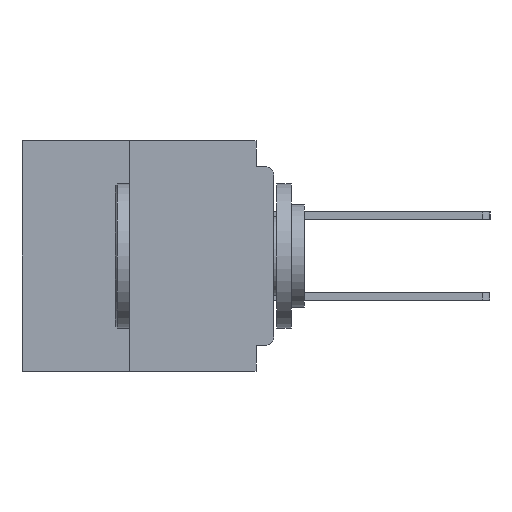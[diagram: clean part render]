
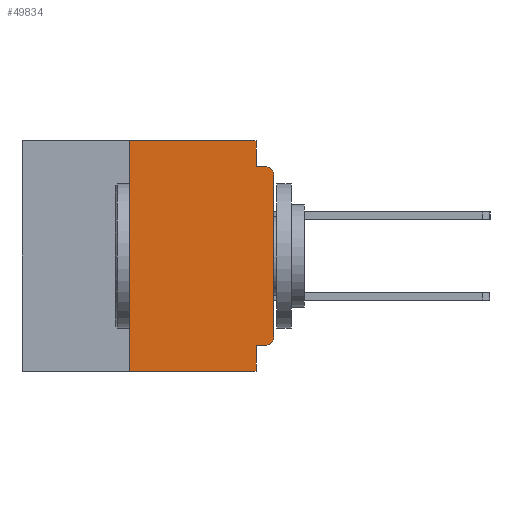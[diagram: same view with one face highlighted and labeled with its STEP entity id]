
A CAD part, left-side view. The second image highlights one B-rep face of the part: STEP entity #49834.
In plain terms, the highlighted planar face has unit normal (-1, 0, 0).
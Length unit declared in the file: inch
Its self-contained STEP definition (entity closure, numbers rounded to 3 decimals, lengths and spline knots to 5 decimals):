
#256 = CARTESIAN_POINT ( 'NONE',  ( 0., 0.031, -0.4 ) ) ;
#563 = LINE ( 'NONE', #10025, #61828 ) ;
#2432 = VECTOR ( 'NONE', #19850, 39.37008 ) ;
#3937 = LINE ( 'NONE', #24716, #2432 ) ;
#4308 = EDGE_CURVE ( 'NONE', #11964, #53646, #60278, .T. ) ;
#4399 = AXIS2_PLACEMENT_3D ( 'NONE', #24030, #57806, #28901 ) ;
#4649 = ORIENTED_EDGE ( 'NONE', *, *, #8739, .F. ) ;
#5130 = DIRECTION ( 'NONE',  ( 0., 1., 0. ) ) ;
#6956 = LINE ( 'NONE', #42299, #56839 ) ;
#6990 = CIRCLE ( 'NONE', #42177, 0.015 ) ;
#8519 = EDGE_CURVE ( 'NONE', #20073, #9102, #41814, .T. ) ;
#8619 = ORIENTED_EDGE ( 'NONE', *, *, #49815, .F. ) ;
#8739 = EDGE_CURVE ( 'NONE', #57338, #20073, #3937, .T. ) ;
#9102 = VERTEX_POINT ( 'NONE', #18107 ) ;
#9490 = DIRECTION ( 'NONE',  ( -1., 0., 0. ) ) ;
#10025 = CARTESIAN_POINT ( 'NONE',  ( 0., 0., -0.355 ) ) ;
#11177 = VERTEX_POINT ( 'NONE', #35930 ) ;
#11964 = VERTEX_POINT ( 'NONE', #17479 ) ;
#13334 = DIRECTION ( 'NONE',  ( 0., -1., 0. ) ) ;
#14566 = ORIENTED_EDGE ( 'NONE', *, *, #35206, .F. ) ;
#14769 = CARTESIAN_POINT ( 'NONE',  ( 0., 0.031, -0.045 ) ) ;
#15001 = CARTESIAN_POINT ( 'NONE',  ( 0., 0.437, -0.4 ) ) ;
#15492 = VECTOR ( 'NONE', #34383, 39.37008 ) ;
#15539 = CARTESIAN_POINT ( 'NONE',  ( 0., 0.25, -0.4 ) ) ;
#16823 = EDGE_CURVE ( 'NONE', #11177, #11964, #23770, .T. ) ;
#17022 = LINE ( 'NONE', #15001, #15492 ) ;
#17479 = CARTESIAN_POINT ( 'NONE',  ( 0., 0., -0.34 ) ) ;
#17970 = EDGE_CURVE ( 'NONE', #47196, #41981, #6956, .T. ) ;
#18107 = CARTESIAN_POINT ( 'NONE',  ( 0., 0.031, 0. ) ) ;
#18958 = PLANE ( 'NONE',  #4399 ) ;
#19850 = DIRECTION ( 'NONE',  ( 0., 0., 1. ) ) ;
#20073 = VERTEX_POINT ( 'NONE', #40100 ) ;
#21197 = ORIENTED_EDGE ( 'NONE', *, *, #4308, .T. ) ;
#22393 = DIRECTION ( 'NONE',  ( -1., 0., 0. ) ) ;
#23007 = LINE ( 'NONE', #47890, #35847 ) ;
#23770 = CIRCLE ( 'NONE', #35963, 0.015 ) ;
#24030 = CARTESIAN_POINT ( 'NONE',  ( 0., 0.437, 0. ) ) ;
#24100 = EDGE_CURVE ( 'NONE', #53646, #46455, #6990, .T. ) ;
#24716 = CARTESIAN_POINT ( 'NONE',  ( 0., 0.25, -0.4 ) ) ;
#24895 = EDGE_LOOP ( 'NONE', ( #21197, #37597, #56532, #8619, #55311, #4649, #39824, #33383, #14566, #56728 ) ) ;
#27067 = DIRECTION ( 'NONE',  ( 0., 0., 1. ) ) ;
#28901 = DIRECTION ( 'NONE',  ( 0., 0., -1. ) ) ;
#29860 = LINE ( 'NONE', #30820, #42701 ) ;
#30196 = CARTESIAN_POINT ( 'NONE',  ( 0., 0.015, -0.045 ) ) ;
#30470 = VECTOR ( 'NONE', #13334, 39.37008 ) ;
#30820 = CARTESIAN_POINT ( 'NONE',  ( 0., 0., -0.045 ) ) ;
#32968 = CARTESIAN_POINT ( 'NONE',  ( 0., 0., -0.06 ) ) ;
#33383 = ORIENTED_EDGE ( 'NONE', *, *, #17970, .F. ) ;
#33504 = DIRECTION ( 'NONE',  ( 0., 0., -1. ) ) ;
#34383 = DIRECTION ( 'NONE',  ( 0., -1., 0. ) ) ;
#35206 = EDGE_CURVE ( 'NONE', #11177, #47196, #563, .T. ) ;
#35847 = VECTOR ( 'NONE', #33504, 39.37008 ) ;
#35930 = CARTESIAN_POINT ( 'NONE',  ( 0., 0.015, -0.355 ) ) ;
#35963 = AXIS2_PLACEMENT_3D ( 'NONE', #38419, #9490, #43281 ) ;
#36775 = VERTEX_POINT ( 'NONE', #14769 ) ;
#37597 = ORIENTED_EDGE ( 'NONE', *, *, #24100, .T. ) ;
#38419 = CARTESIAN_POINT ( 'NONE',  ( 0., 0.015, -0.34 ) ) ;
#39824 = ORIENTED_EDGE ( 'NONE', *, *, #56652, .T. ) ;
#40100 = CARTESIAN_POINT ( 'NONE',  ( 0., 0.25, 0. ) ) ;
#40868 = CARTESIAN_POINT ( 'NONE',  ( 0., 0.031, -0.355 ) ) ;
#41814 = LINE ( 'NONE', #42266, #30470 ) ;
#41981 = VERTEX_POINT ( 'NONE', #256 ) ;
#42177 = AXIS2_PLACEMENT_3D ( 'NONE', #51327, #22393, #56187 ) ;
#42266 = CARTESIAN_POINT ( 'NONE',  ( 0., 0.437, 0. ) ) ;
#42299 = CARTESIAN_POINT ( 'NONE',  ( 0., 0.031, -0.4 ) ) ;
#42701 = VECTOR ( 'NONE', #59752, 39.37008 ) ;
#43281 = DIRECTION ( 'NONE',  ( 0., 0., -1. ) ) ;
#46455 = VERTEX_POINT ( 'NONE', #30196 ) ;
#47185 = FACE_OUTER_BOUND ( 'NONE', #24895, .T. ) ;
#47196 = VERTEX_POINT ( 'NONE', #40868 ) ;
#47431 = VECTOR ( 'NONE', #27067, 39.37008 ) ;
#47890 = CARTESIAN_POINT ( 'NONE',  ( 0., 0.031, 0. ) ) ;
#49448 = EDGE_CURVE ( 'NONE', #36775, #46455, #29860, .T. ) ;
#49815 = EDGE_CURVE ( 'NONE', #9102, #36775, #23007, .T. ) ;
#49834 = ADVANCED_FACE ( 'NONE', ( #47185 ), #18958, .F. ) ;
#51123 = CARTESIAN_POINT ( 'NONE',  ( 0., 0., 0. ) ) ;
#51327 = CARTESIAN_POINT ( 'NONE',  ( 0., 0.015, -0.06 ) ) ;
#53646 = VERTEX_POINT ( 'NONE', #32968 ) ;
#55311 = ORIENTED_EDGE ( 'NONE', *, *, #8519, .F. ) ;
#56187 = DIRECTION ( 'NONE',  ( 0., 0., -1. ) ) ;
#56532 = ORIENTED_EDGE ( 'NONE', *, *, #49448, .F. ) ;
#56652 = EDGE_CURVE ( 'NONE', #57338, #41981, #17022, .T. ) ;
#56728 = ORIENTED_EDGE ( 'NONE', *, *, #16823, .T. ) ;
#56839 = VECTOR ( 'NONE', #61725, 39.37008 ) ;
#57338 = VERTEX_POINT ( 'NONE', #15539 ) ;
#57806 = DIRECTION ( 'NONE',  ( 1., 0., 0. ) ) ;
#59752 = DIRECTION ( 'NONE',  ( 0., -1., 0. ) ) ;
#60278 = LINE ( 'NONE', #51123, #47431 ) ;
#61725 = DIRECTION ( 'NONE',  ( 0., 0., -1. ) ) ;
#61828 = VECTOR ( 'NONE', #5130, 39.37008 ) ;
